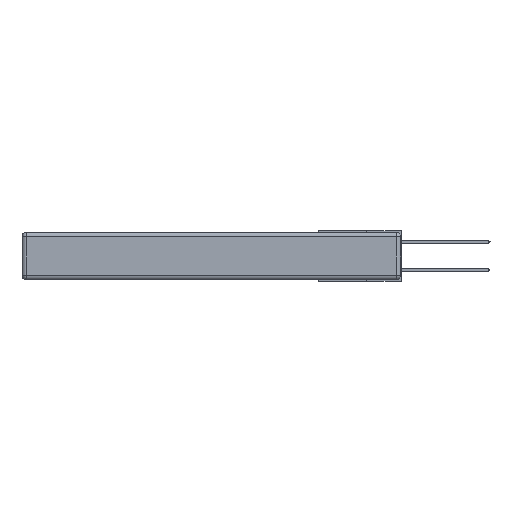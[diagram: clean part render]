
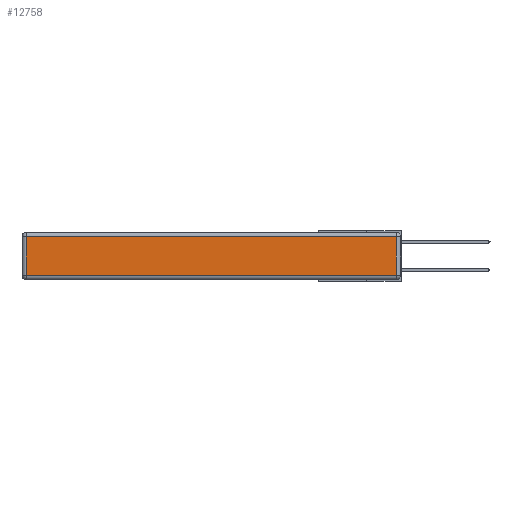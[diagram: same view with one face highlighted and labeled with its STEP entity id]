
A CAD part, left-side view. The second image highlights one B-rep face of the part: STEP entity #12758.
In plain terms, the highlighted planar face has unit normal (-1, 0, 0).
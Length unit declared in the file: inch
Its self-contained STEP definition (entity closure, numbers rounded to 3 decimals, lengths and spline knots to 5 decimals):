
#63 = LINE ( 'NONE', #8132, #11031 ) ;
#795 = AXIS2_PLACEMENT_3D ( 'NONE', #5416, #14501, #893 ) ;
#893 = DIRECTION ( 'NONE',  ( 0., 0., 1. ) ) ;
#1204 = EDGE_CURVE ( 'NONE', #14652, #11170, #12602, .T. ) ;
#1235 = VERTEX_POINT ( 'NONE', #4400 ) ;
#2269 = EDGE_CURVE ( 'NONE', #1235, #11616, #6023, .T. ) ;
#3682 = EDGE_CURVE ( 'NONE', #11616, #14652, #9731, .T. ) ;
#4014 = FACE_OUTER_BOUND ( 'NONE', #13030, .T. ) ;
#4169 = ORIENTED_EDGE ( 'NONE', *, *, #3682, .T. ) ;
#4400 = CARTESIAN_POINT ( 'NONE',  ( 0., 0.03, -0.313 ) ) ;
#4797 = CARTESIAN_POINT ( 'NONE',  ( 0., 2.72, -0.313 ) ) ;
#5416 = CARTESIAN_POINT ( 'NONE',  ( 0., 0., -0.343 ) ) ;
#5792 = ORIENTED_EDGE ( 'NONE', *, *, #1204, .T. ) ;
#6023 = LINE ( 'NONE', #6976, #11701 ) ;
#6879 = VECTOR ( 'NONE', #12403, 39.37008 ) ;
#6976 = CARTESIAN_POINT ( 'NONE',  ( 0., 0.03, -0.343 ) ) ;
#8132 = CARTESIAN_POINT ( 'NONE',  ( 0., 0., -0.313 ) ) ;
#8459 = CARTESIAN_POINT ( 'NONE',  ( 0., 2.75, -0.03 ) ) ;
#8886 = VECTOR ( 'NONE', #12106, 39.37008 ) ;
#9273 = DIRECTION ( 'NONE',  ( 0., -1., 0. ) ) ;
#9508 = EDGE_CURVE ( 'NONE', #11170, #1235, #63, .T. ) ;
#9731 = LINE ( 'NONE', #8459, #6879 ) ;
#11031 = VECTOR ( 'NONE', #9273, 39.37008 ) ;
#11170 = VERTEX_POINT ( 'NONE', #4797 ) ;
#11616 = VERTEX_POINT ( 'NONE', #14577 ) ;
#11701 = VECTOR ( 'NONE', #13942, 39.37008 ) ;
#12106 = DIRECTION ( 'NONE',  ( 0., 0., -1. ) ) ;
#12207 = PLANE ( 'NONE',  #795 ) ;
#12403 = DIRECTION ( 'NONE',  ( 0., 1., 0. ) ) ;
#12602 = LINE ( 'NONE', #13282, #8886 ) ;
#12758 = ADVANCED_FACE ( 'NONE', ( #4014 ), #12207, .T. ) ;
#12960 = ORIENTED_EDGE ( 'NONE', *, *, #2269, .T. ) ;
#13030 = EDGE_LOOP ( 'NONE', ( #13801, #12960, #4169, #5792 ) ) ;
#13282 = CARTESIAN_POINT ( 'NONE',  ( 0., 2.72, -0.343 ) ) ;
#13801 = ORIENTED_EDGE ( 'NONE', *, *, #9508, .T. ) ;
#13942 = DIRECTION ( 'NONE',  ( 0., 0., 1. ) ) ;
#14184 = CARTESIAN_POINT ( 'NONE',  ( 0., 2.72, -0.03 ) ) ;
#14501 = DIRECTION ( 'NONE',  ( -1., 0., 0. ) ) ;
#14577 = CARTESIAN_POINT ( 'NONE',  ( 0., 0.03, -0.03 ) ) ;
#14652 = VERTEX_POINT ( 'NONE', #14184 ) ;
